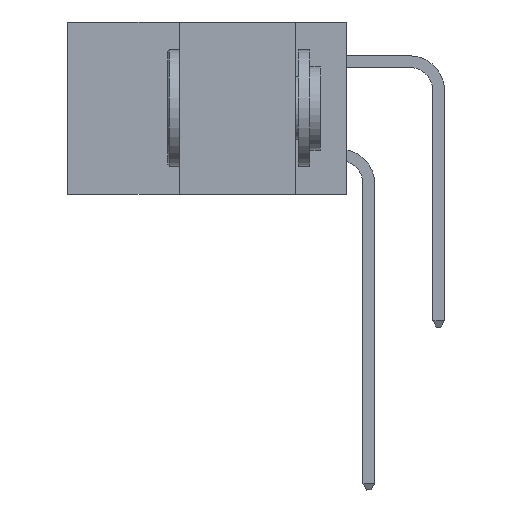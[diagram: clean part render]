
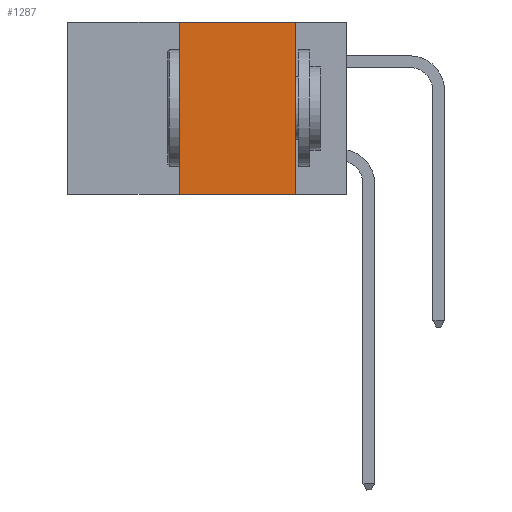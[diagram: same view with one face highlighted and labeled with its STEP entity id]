
A CAD part, left-side view. The second image highlights one B-rep face of the part: STEP entity #1287.
In plain terms, the highlighted planar face has unit normal (-1, 0, 0).
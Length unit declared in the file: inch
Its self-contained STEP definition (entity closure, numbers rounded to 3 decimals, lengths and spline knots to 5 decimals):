
#495 = LINE ( 'NONE', #22876, #15817 ) ;
#870 = VERTEX_POINT ( 'NONE', #17159 ) ;
#1287 = ADVANCED_FACE ( 'NONE', ( #30776 ), #8785, .F. ) ;
#4009 = CARTESIAN_POINT ( 'NONE',  ( 0., 0.6, 0. ) ) ;
#5153 = CARTESIAN_POINT ( 'NONE',  ( 0., 0.6, -0.37 ) ) ;
#5696 = VECTOR ( 'NONE', #12507, 39.37008 ) ;
#6092 = CARTESIAN_POINT ( 'NONE',  ( 0., 0.36, 0. ) ) ;
#6844 = DIRECTION ( 'NONE',  ( 0., -1., 0. ) ) ;
#7346 = LINE ( 'NONE', #5153, #25536 ) ;
#8708 = EDGE_LOOP ( 'NONE', ( #19457, #28607, #16412, #22691 ) ) ;
#8785 = PLANE ( 'NONE',  #14963 ) ;
#9984 = VERTEX_POINT ( 'NONE', #10840 ) ;
#10840 = CARTESIAN_POINT ( 'NONE',  ( 0., 0.36, -0.37 ) ) ;
#10898 = LINE ( 'NONE', #20497, #5696 ) ;
#12507 = DIRECTION ( 'NONE',  ( 0., 0., -1. ) ) ;
#14579 = CARTESIAN_POINT ( 'NONE',  ( 0., 0.11, -0.37 ) ) ;
#14963 = AXIS2_PLACEMENT_3D ( 'NONE', #32049, #24375, #31702 ) ;
#15817 = VECTOR ( 'NONE', #17883, 39.37008 ) ;
#16412 = ORIENTED_EDGE ( 'NONE', *, *, #30304, .F. ) ;
#17159 = CARTESIAN_POINT ( 'NONE',  ( 0., 0.11, 0. ) ) ;
#17883 = DIRECTION ( 'NONE',  ( 0., 0., 1. ) ) ;
#19362 = EDGE_CURVE ( 'NONE', #870, #31356, #10898, .T. ) ;
#19457 = ORIENTED_EDGE ( 'NONE', *, *, #19362, .F. ) ;
#20497 = CARTESIAN_POINT ( 'NONE',  ( 0., 0.11, 0. ) ) ;
#20742 = DIRECTION ( 'NONE',  ( 0., -1., 0. ) ) ;
#21163 = LINE ( 'NONE', #4009, #24752 ) ;
#22691 = ORIENTED_EDGE ( 'NONE', *, *, #30351, .T. ) ;
#22876 = CARTESIAN_POINT ( 'NONE',  ( 0., 0.36, 0. ) ) ;
#24375 = DIRECTION ( 'NONE',  ( 1., 0., 0. ) ) ;
#24479 = VERTEX_POINT ( 'NONE', #6092 ) ;
#24752 = VECTOR ( 'NONE', #6844, 39.37008 ) ;
#25536 = VECTOR ( 'NONE', #20742, 39.37008 ) ;
#28607 = ORIENTED_EDGE ( 'NONE', *, *, #30174, .F. ) ;
#30174 = EDGE_CURVE ( 'NONE', #24479, #870, #21163, .T. ) ;
#30304 = EDGE_CURVE ( 'NONE', #9984, #24479, #495, .T. ) ;
#30351 = EDGE_CURVE ( 'NONE', #9984, #31356, #7346, .T. ) ;
#30776 = FACE_OUTER_BOUND ( 'NONE', #8708, .T. ) ;
#31356 = VERTEX_POINT ( 'NONE', #14579 ) ;
#31702 = DIRECTION ( 'NONE',  ( 0., 0., -1. ) ) ;
#32049 = CARTESIAN_POINT ( 'NONE',  ( 0., 0.6, 0. ) ) ;
